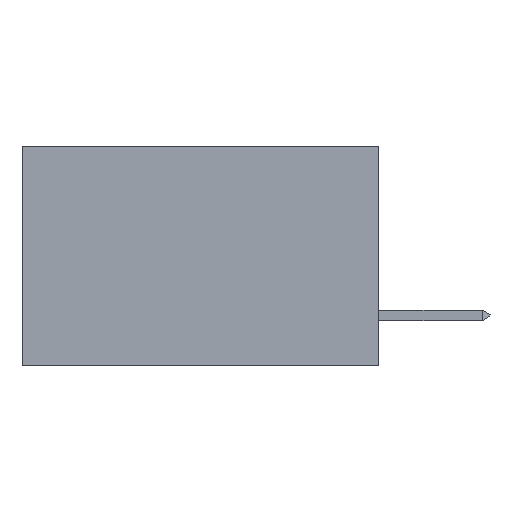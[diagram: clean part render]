
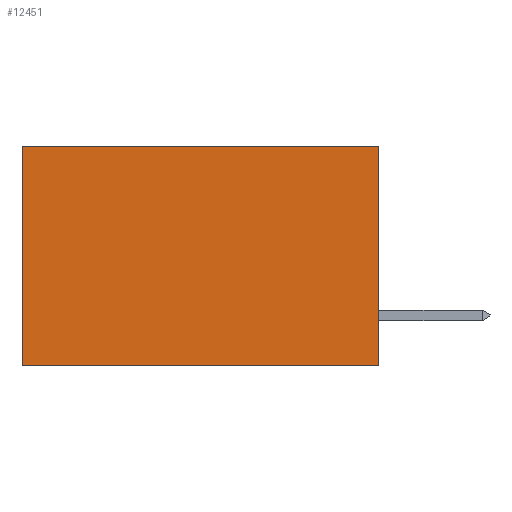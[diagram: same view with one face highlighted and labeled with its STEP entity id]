
A CAD part, left-side view. The second image highlights one B-rep face of the part: STEP entity #12451.
In plain terms, the highlighted planar face has unit normal (-1, 0, 0).
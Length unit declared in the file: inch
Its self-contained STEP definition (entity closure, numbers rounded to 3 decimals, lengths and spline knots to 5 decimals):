
#377 = VECTOR ( 'NONE', #8864, 39.37008 ) ;
#998 = VERTEX_POINT ( 'NONE', #5395 ) ;
#1130 = CARTESIAN_POINT ( 'NONE',  ( 0.2615, 0., -0.37 ) ) ;
#3168 = LINE ( 'NONE', #22961, #6930 ) ;
#5212 = DIRECTION ( 'NONE',  ( 0., 1., 0. ) ) ;
#5395 = CARTESIAN_POINT ( 'NONE',  ( 0.2615, 0.6, 0. ) ) ;
#5963 = ORIENTED_EDGE ( 'NONE', *, *, #6702, .F. ) ;
#6407 = ORIENTED_EDGE ( 'NONE', *, *, #22413, .T. ) ;
#6702 = EDGE_CURVE ( 'NONE', #21595, #22617, #18649, .T. ) ;
#6930 = VECTOR ( 'NONE', #7630, 39.37008 ) ;
#7630 = DIRECTION ( 'NONE',  ( 0., 1., 0. ) ) ;
#7848 = PLANE ( 'NONE',  #18550 ) ;
#8864 = DIRECTION ( 'NONE',  ( 0., 0., -1. ) ) ;
#10628 = LINE ( 'NONE', #10877, #377 ) ;
#10859 = VECTOR ( 'NONE', #5212, 39.37008 ) ;
#10877 = CARTESIAN_POINT ( 'NONE',  ( 0.2615, 0., -0.37 ) ) ;
#11150 = CARTESIAN_POINT ( 'NONE',  ( 0.2615, 0., -0.37 ) ) ;
#11513 = DIRECTION ( 'NONE',  ( 1., 0., 0. ) ) ;
#11637 = CARTESIAN_POINT ( 'NONE',  ( 0.2615, 0., -0.37 ) ) ;
#12451 = ADVANCED_FACE ( 'NONE', ( #19498 ), #7848, .F. ) ;
#12503 = LINE ( 'NONE', #22510, #22393 ) ;
#12728 = EDGE_LOOP ( 'NONE', ( #6407, #5963, #15803, #16716 ) ) ;
#14781 = DIRECTION ( 'NONE',  ( 0., 0., -1. ) ) ;
#15803 = ORIENTED_EDGE ( 'NONE', *, *, #16706, .F. ) ;
#16706 = EDGE_CURVE ( 'NONE', #21486, #21595, #10628, .T. ) ;
#16716 = ORIENTED_EDGE ( 'NONE', *, *, #18243, .T. ) ;
#18243 = EDGE_CURVE ( 'NONE', #21486, #998, #3168, .T. ) ;
#18550 = AXIS2_PLACEMENT_3D ( 'NONE', #11637, #11513, #19256 ) ;
#18649 = LINE ( 'NONE', #1130, #10859 ) ;
#19256 = DIRECTION ( 'NONE',  ( 0., 0., -1. ) ) ;
#19498 = FACE_OUTER_BOUND ( 'NONE', #12728, .T. ) ;
#21130 = CARTESIAN_POINT ( 'NONE',  ( 0.2615, 0.6, -0.37 ) ) ;
#21486 = VERTEX_POINT ( 'NONE', #22570 ) ;
#21595 = VERTEX_POINT ( 'NONE', #11150 ) ;
#22393 = VECTOR ( 'NONE', #14781, 39.37008 ) ;
#22413 = EDGE_CURVE ( 'NONE', #998, #22617, #12503, .T. ) ;
#22510 = CARTESIAN_POINT ( 'NONE',  ( 0.2615, 0.6, -0.37 ) ) ;
#22570 = CARTESIAN_POINT ( 'NONE',  ( 0.2615, 0., 0. ) ) ;
#22617 = VERTEX_POINT ( 'NONE', #21130 ) ;
#22961 = CARTESIAN_POINT ( 'NONE',  ( 0.2615, 0., 0. ) ) ;
